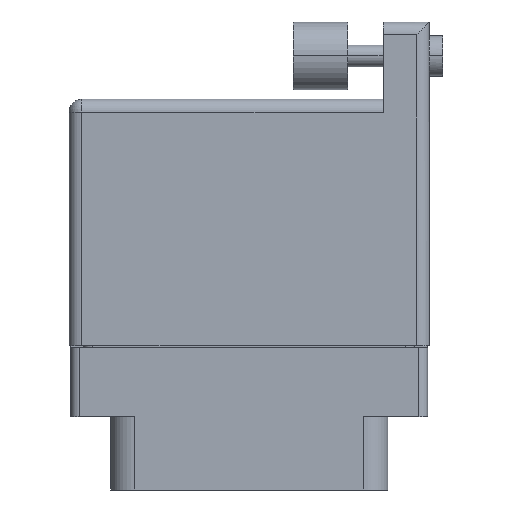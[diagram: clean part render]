
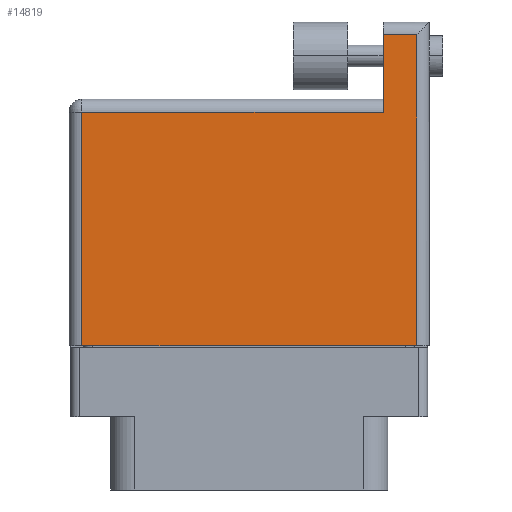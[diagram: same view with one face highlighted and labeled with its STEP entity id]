
A CAD part, front view. The second image highlights one B-rep face of the part: STEP entity #14819.
In plain terms, the highlighted face is planar.
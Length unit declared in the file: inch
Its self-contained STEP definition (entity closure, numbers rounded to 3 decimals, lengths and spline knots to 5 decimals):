
#765 = ORIENTED_EDGE ( 'NONE', *, *, #21099, .T. ) ;
#1046 = VECTOR ( 'NONE', #3972, 39.37008 ) ;
#1934 = DIRECTION ( 'NONE',  ( -1., 0., 0. ) ) ;
#2767 = CARTESIAN_POINT ( 'NONE',  ( -0.6625, -0.1, 0.3575 ) ) ;
#3248 = VERTEX_POINT ( 'NONE', #16114 ) ;
#3615 = LINE ( 'NONE', #11655, #17558 ) ;
#3719 = LINE ( 'NONE', #11754, #1046 ) ;
#3972 = DIRECTION ( 'NONE',  ( 0., 1., 0. ) ) ;
#5700 = ORIENTED_EDGE ( 'NONE', *, *, #15690, .T. ) ;
#5791 = EDGE_CURVE ( 'NONE', #23661, #8935, #20235, .T. ) ;
#6019 = CARTESIAN_POINT ( 'NONE',  ( 0.4925, 0.759, 0.3575 ) ) ;
#6408 = FACE_OUTER_BOUND ( 'NONE', #12246, .T. ) ;
#6913 = EDGE_CURVE ( 'NONE', #3248, #15986, #9203, .T. ) ;
#7804 = LINE ( 'NONE', #14116, #24246 ) ;
#7867 = VECTOR ( 'NONE', #12360, 39.37008 ) ;
#7884 = VECTOR ( 'NONE', #14877, 39.37008 ) ;
#8124 = ORIENTED_EDGE ( 'NONE', *, *, #6913, .T. ) ;
#8935 = VERTEX_POINT ( 'NONE', #23226 ) ;
#9072 = AXIS2_PLACEMENT_3D ( 'NONE', #20360, #24047, #1934 ) ;
#9203 = LINE ( 'NONE', #2767, #7884 ) ;
#10245 = CARTESIAN_POINT ( 'NONE',  ( -0.6625, 0.759, 0.3575 ) ) ;
#11130 = EDGE_CURVE ( 'NONE', #15986, #15998, #3719, .T. ) ;
#11300 = VERTEX_POINT ( 'NONE', #17213 ) ;
#11655 = CARTESIAN_POINT ( 'NONE',  ( 0.4925, 1.043, 0.3575 ) ) ;
#11754 = CARTESIAN_POINT ( 'NONE',  ( 0.6155, 1.09, 0.3575 ) ) ;
#12246 = EDGE_LOOP ( 'NONE', ( #8124, #19360, #765, #16370, #20721, #5700 ) ) ;
#12360 = DIRECTION ( 'NONE',  ( -1., 0., 0. ) ) ;
#13720 = LINE ( 'NONE', #21733, #20932 ) ;
#13871 = DIRECTION ( 'NONE',  ( -1., 0., 0. ) ) ;
#14116 = CARTESIAN_POINT ( 'NONE',  ( -0.6155, -0.1, 0.3575 ) ) ;
#14819 = ADVANCED_FACE ( 'NONE', ( #6408 ), #20496, .F. ) ;
#14877 = DIRECTION ( 'NONE',  ( 1., 0., 0. ) ) ;
#15690 = EDGE_CURVE ( 'NONE', #8935, #3248, #7804, .T. ) ;
#15821 = DIRECTION ( 'NONE',  ( 0., -1., 0. ) ) ;
#15986 = VERTEX_POINT ( 'NONE', #17511 ) ;
#15998 = VERTEX_POINT ( 'NONE', #25533 ) ;
#16114 = CARTESIAN_POINT ( 'NONE',  ( -0.6155, -0.1, 0.3575 ) ) ;
#16370 = ORIENTED_EDGE ( 'NONE', *, *, #21579, .T. ) ;
#17213 = CARTESIAN_POINT ( 'NONE',  ( 0.4925, 1.043, 0.3575 ) ) ;
#17511 = CARTESIAN_POINT ( 'NONE',  ( 0.6155, -0.1, 0.3575 ) ) ;
#17558 = VECTOR ( 'NONE', #13871, 39.37008 ) ;
#19360 = ORIENTED_EDGE ( 'NONE', *, *, #11130, .T. ) ;
#20235 = LINE ( 'NONE', #10245, #7867 ) ;
#20360 = CARTESIAN_POINT ( 'NONE',  ( -0.6625, 0.806, 0.3575 ) ) ;
#20496 = PLANE ( 'NONE',  #9072 ) ;
#20721 = ORIENTED_EDGE ( 'NONE', *, *, #5791, .T. ) ;
#20932 = VECTOR ( 'NONE', #15821, 39.37008 ) ;
#21099 = EDGE_CURVE ( 'NONE', #15998, #11300, #3615, .T. ) ;
#21579 = EDGE_CURVE ( 'NONE', #11300, #23661, #13720, .T. ) ;
#21733 = CARTESIAN_POINT ( 'NONE',  ( 0.4925, 1.09, 0.3575 ) ) ;
#21865 = DIRECTION ( 'NONE',  ( 0., -1., 0. ) ) ;
#23226 = CARTESIAN_POINT ( 'NONE',  ( -0.6155, 0.759, 0.3575 ) ) ;
#23661 = VERTEX_POINT ( 'NONE', #6019 ) ;
#24047 = DIRECTION ( 'NONE',  ( 0., 0., -1. ) ) ;
#24246 = VECTOR ( 'NONE', #21865, 39.37008 ) ;
#25533 = CARTESIAN_POINT ( 'NONE',  ( 0.6155, 1.043, 0.3575 ) ) ;
